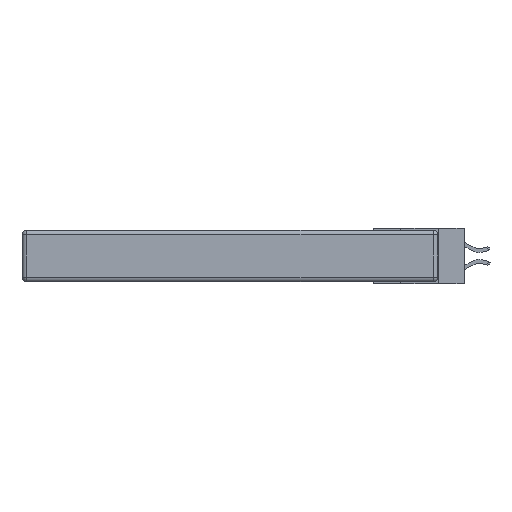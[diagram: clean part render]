
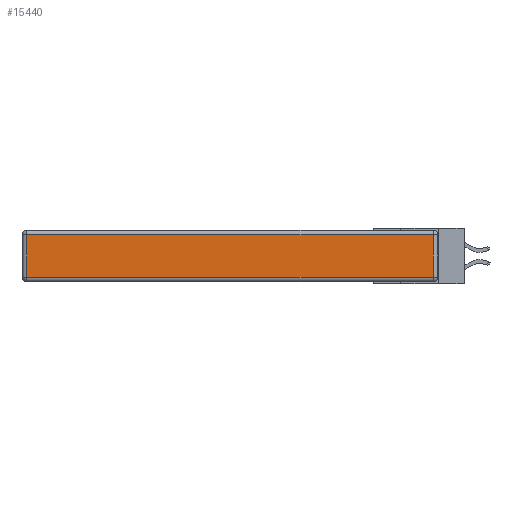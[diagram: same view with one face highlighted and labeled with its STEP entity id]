
A CAD part, left-side view. The second image highlights one B-rep face of the part: STEP entity #15440.
In plain terms, the highlighted planar face has unit normal (-1, 0, 0).
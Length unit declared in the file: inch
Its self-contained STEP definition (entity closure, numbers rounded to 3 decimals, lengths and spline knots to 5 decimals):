
#937 = DIRECTION ( 'NONE',  ( 0., 0., -1. ) ) ;
#1004 = DIRECTION ( 'NONE',  ( 0., 0., 1. ) ) ;
#1430 = VERTEX_POINT ( 'NONE', #20213 ) ;
#1967 = EDGE_CURVE ( 'NONE', #33587, #10391, #22905, .T. ) ;
#2636 = ORIENTED_EDGE ( 'NONE', *, *, #1967, .T. ) ;
#2883 = EDGE_CURVE ( 'NONE', #29531, #1430, #33141, .T. ) ;
#2913 = LINE ( 'NONE', #26385, #32884 ) ;
#5976 = DIRECTION ( 'NONE',  ( 0., 1., 0. ) ) ;
#7282 = EDGE_CURVE ( 'NONE', #10391, #29531, #8113, .T. ) ;
#8113 = LINE ( 'NONE', #16926, #24775 ) ;
#10391 = VERTEX_POINT ( 'NONE', #23460 ) ;
#11173 = DIRECTION ( 'NONE',  ( 0., 0., 1. ) ) ;
#13254 = ORIENTED_EDGE ( 'NONE', *, *, #26429, .T. ) ;
#14223 = CARTESIAN_POINT ( 'NONE',  ( 0., 0.03, -0.343 ) ) ;
#15440 = ADVANCED_FACE ( 'NONE', ( #16192 ), #19087, .T. ) ;
#15804 = VECTOR ( 'NONE', #1004, 39.37008 ) ;
#16192 = FACE_OUTER_BOUND ( 'NONE', #23434, .T. ) ;
#16926 = CARTESIAN_POINT ( 'NONE',  ( 0., 2.75, -0.03 ) ) ;
#18468 = DIRECTION ( 'NONE',  ( 0., -1., 0. ) ) ;
#18713 = CARTESIAN_POINT ( 'NONE',  ( 0., 0.03, -0.313 ) ) ;
#19045 = VECTOR ( 'NONE', #937, 39.37008 ) ;
#19087 = PLANE ( 'NONE',  #31832 ) ;
#20213 = CARTESIAN_POINT ( 'NONE',  ( 0., 2.72, -0.313 ) ) ;
#21783 = CARTESIAN_POINT ( 'NONE',  ( 0., 0., -0.343 ) ) ;
#22905 = LINE ( 'NONE', #14223, #15804 ) ;
#23434 = EDGE_LOOP ( 'NONE', ( #13254, #2636, #23870, #27719 ) ) ;
#23460 = CARTESIAN_POINT ( 'NONE',  ( 0., 0.03, -0.03 ) ) ;
#23870 = ORIENTED_EDGE ( 'NONE', *, *, #7282, .T. ) ;
#23872 = CARTESIAN_POINT ( 'NONE',  ( 0., 2.72, -0.03 ) ) ;
#24775 = VECTOR ( 'NONE', #5976, 39.37008 ) ;
#24795 = DIRECTION ( 'NONE',  ( -1., 0., 0. ) ) ;
#26385 = CARTESIAN_POINT ( 'NONE',  ( 0., 0., -0.313 ) ) ;
#26429 = EDGE_CURVE ( 'NONE', #1430, #33587, #2913, .T. ) ;
#27719 = ORIENTED_EDGE ( 'NONE', *, *, #2883, .T. ) ;
#29531 = VERTEX_POINT ( 'NONE', #23872 ) ;
#30199 = CARTESIAN_POINT ( 'NONE',  ( 0., 2.72, -0.343 ) ) ;
#31832 = AXIS2_PLACEMENT_3D ( 'NONE', #21783, #24795, #11173 ) ;
#32884 = VECTOR ( 'NONE', #18468, 39.37008 ) ;
#33141 = LINE ( 'NONE', #30199, #19045 ) ;
#33587 = VERTEX_POINT ( 'NONE', #18713 ) ;
